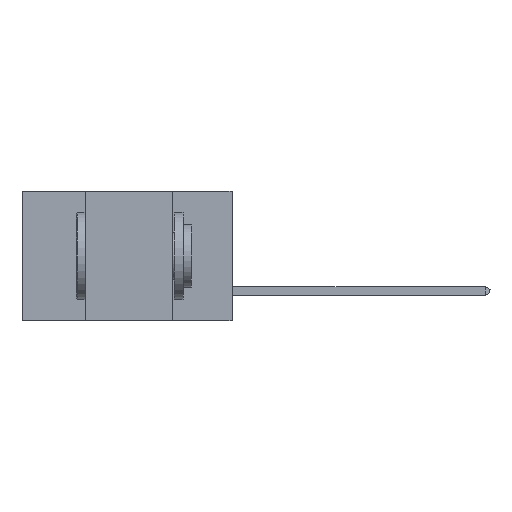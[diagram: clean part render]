
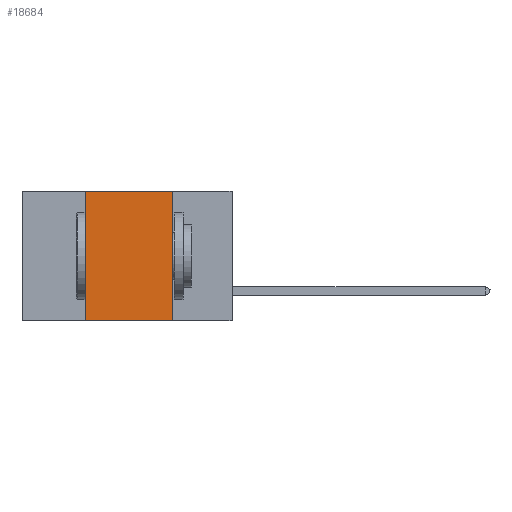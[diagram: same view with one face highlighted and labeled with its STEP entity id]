
A CAD part, left-side view. The second image highlights one B-rep face of the part: STEP entity #18684.
In plain terms, the highlighted planar face has unit normal (-1, 0, 0).
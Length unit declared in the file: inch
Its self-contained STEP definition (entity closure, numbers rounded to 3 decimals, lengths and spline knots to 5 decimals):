
#129 = CARTESIAN_POINT ( 'NONE',  ( 0., 0.6, 0. ) ) ;
#505 = LINE ( 'NONE', #13010, #23595 ) ;
#550 = LINE ( 'NONE', #8338, #7129 ) ;
#1802 = ORIENTED_EDGE ( 'NONE', *, *, #20988, .F. ) ;
#1865 = LINE ( 'NONE', #25473, #22563 ) ;
#2024 = VERTEX_POINT ( 'NONE', #17479 ) ;
#2607 = CARTESIAN_POINT ( 'NONE',  ( 0., 0.17, 0. ) ) ;
#4180 = DIRECTION ( 'NONE',  ( 0., -1., 0. ) ) ;
#4805 = EDGE_LOOP ( 'NONE', ( #20439, #1802, #24295, #22540 ) ) ;
#5671 = AXIS2_PLACEMENT_3D ( 'NONE', #129, #19167, #17352 ) ;
#6523 = DIRECTION ( 'NONE',  ( 0., 0., -1. ) ) ;
#7129 = VECTOR ( 'NONE', #14453, 39.37008 ) ;
#8121 = VERTEX_POINT ( 'NONE', #24529 ) ;
#8338 = CARTESIAN_POINT ( 'NONE',  ( 0., 0.42, 0. ) ) ;
#11070 = DIRECTION ( 'NONE',  ( 0., -1., 0. ) ) ;
#12624 = LINE ( 'NONE', #23188, #16637 ) ;
#13010 = CARTESIAN_POINT ( 'NONE',  ( 0., 0.6, -0.37 ) ) ;
#13700 = VERTEX_POINT ( 'NONE', #27050 ) ;
#14415 = FACE_OUTER_BOUND ( 'NONE', #4805, .T. ) ;
#14453 = DIRECTION ( 'NONE',  ( 0., 0., 1. ) ) ;
#15041 = PLANE ( 'NONE',  #5671 ) ;
#16637 = VECTOR ( 'NONE', #11070, 39.37008 ) ;
#17352 = DIRECTION ( 'NONE',  ( 0., 0., -1. ) ) ;
#17479 = CARTESIAN_POINT ( 'NONE',  ( 0., 0.42, 0. ) ) ;
#18609 = EDGE_CURVE ( 'NONE', #13700, #8121, #505, .T. ) ;
#18684 = ADVANCED_FACE ( 'NONE', ( #14415 ), #15041, .F. ) ;
#19167 = DIRECTION ( 'NONE',  ( 1., 0., 0. ) ) ;
#20439 = ORIENTED_EDGE ( 'NONE', *, *, #26002, .F. ) ;
#20978 = VERTEX_POINT ( 'NONE', #2607 ) ;
#20988 = EDGE_CURVE ( 'NONE', #2024, #20978, #12624, .T. ) ;
#22540 = ORIENTED_EDGE ( 'NONE', *, *, #18609, .T. ) ;
#22563 = VECTOR ( 'NONE', #6523, 39.37008 ) ;
#23188 = CARTESIAN_POINT ( 'NONE',  ( 0., 0.6, 0. ) ) ;
#23595 = VECTOR ( 'NONE', #4180, 39.37008 ) ;
#24295 = ORIENTED_EDGE ( 'NONE', *, *, #24596, .F. ) ;
#24529 = CARTESIAN_POINT ( 'NONE',  ( 0., 0.17, -0.37 ) ) ;
#24596 = EDGE_CURVE ( 'NONE', #13700, #2024, #550, .T. ) ;
#25473 = CARTESIAN_POINT ( 'NONE',  ( 0., 0.17, 0. ) ) ;
#26002 = EDGE_CURVE ( 'NONE', #20978, #8121, #1865, .T. ) ;
#27050 = CARTESIAN_POINT ( 'NONE',  ( 0., 0.42, -0.37 ) ) ;
